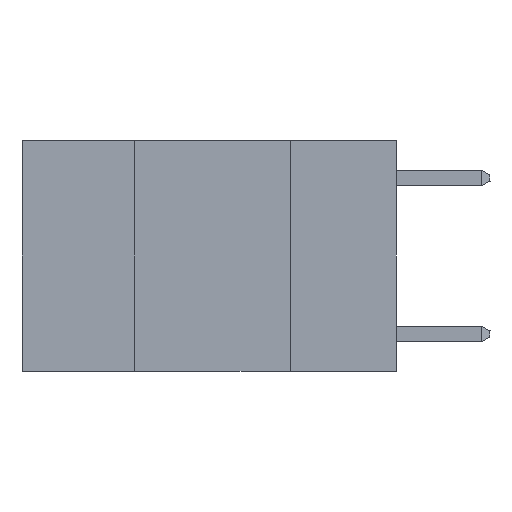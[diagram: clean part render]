
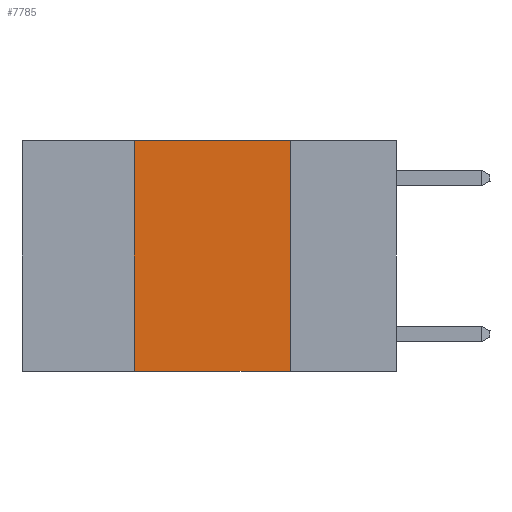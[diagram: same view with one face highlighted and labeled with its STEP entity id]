
A CAD part, left-side view. The second image highlights one B-rep face of the part: STEP entity #7785.
In plain terms, the highlighted planar face has unit normal (-1, 0, 0).
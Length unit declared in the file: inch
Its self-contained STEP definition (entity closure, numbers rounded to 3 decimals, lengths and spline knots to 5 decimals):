
#17 = VERTEX_POINT ( 'NONE', #8199 ) ;
#267 = PLANE ( 'NONE',  #1084 ) ;
#646 = EDGE_CURVE ( 'NONE', #10710, #13058, #12916, .T. ) ;
#807 = CARTESIAN_POINT ( 'NONE',  ( 0., 0.17, 0. ) ) ;
#955 = VECTOR ( 'NONE', #2615, 39.37008 ) ;
#989 = EDGE_CURVE ( 'NONE', #13058, #6762, #6658, .T. ) ;
#1084 = AXIS2_PLACEMENT_3D ( 'NONE', #8690, #9855, #2720 ) ;
#2025 = DIRECTION ( 'NONE',  ( 0., 0., -1. ) ) ;
#2289 = EDGE_CURVE ( 'NONE', #10710, #17, #6254, .T. ) ;
#2615 = DIRECTION ( 'NONE',  ( 0., -1., 0. ) ) ;
#2720 = DIRECTION ( 'NONE',  ( 0., 0., -1. ) ) ;
#2868 = VECTOR ( 'NONE', #7105, 39.37008 ) ;
#3049 = FACE_OUTER_BOUND ( 'NONE', #4966, .T. ) ;
#3768 = VECTOR ( 'NONE', #9450, 39.37008 ) ;
#3850 = CARTESIAN_POINT ( 'NONE',  ( 0., 0.42, 0. ) ) ;
#4619 = CARTESIAN_POINT ( 'NONE',  ( 0., 0.6, -0.37 ) ) ;
#4966 = EDGE_LOOP ( 'NONE', ( #12845, #11351, #13633, #12426 ) ) ;
#6254 = LINE ( 'NONE', #4619, #955 ) ;
#6658 = LINE ( 'NONE', #10931, #2868 ) ;
#6762 = VERTEX_POINT ( 'NONE', #9344 ) ;
#6813 = VECTOR ( 'NONE', #2025, 39.37008 ) ;
#7032 = CARTESIAN_POINT ( 'NONE',  ( 0., 0.42, -0.37 ) ) ;
#7105 = DIRECTION ( 'NONE',  ( 0., -1., 0. ) ) ;
#7785 = ADVANCED_FACE ( 'NONE', ( #3049 ), #267, .F. ) ;
#8092 = CARTESIAN_POINT ( 'NONE',  ( 0., 0.42, 0. ) ) ;
#8199 = CARTESIAN_POINT ( 'NONE',  ( 0., 0.17, -0.37 ) ) ;
#8690 = CARTESIAN_POINT ( 'NONE',  ( 0., 0.6, 0. ) ) ;
#8698 = EDGE_CURVE ( 'NONE', #6762, #17, #13298, .T. ) ;
#9344 = CARTESIAN_POINT ( 'NONE',  ( 0., 0.17, 0. ) ) ;
#9450 = DIRECTION ( 'NONE',  ( 0., 0., 1. ) ) ;
#9855 = DIRECTION ( 'NONE',  ( 1., 0., 0. ) ) ;
#10710 = VERTEX_POINT ( 'NONE', #7032 ) ;
#10931 = CARTESIAN_POINT ( 'NONE',  ( 0., 0.6, 0. ) ) ;
#11351 = ORIENTED_EDGE ( 'NONE', *, *, #989, .F. ) ;
#12426 = ORIENTED_EDGE ( 'NONE', *, *, #2289, .T. ) ;
#12845 = ORIENTED_EDGE ( 'NONE', *, *, #8698, .F. ) ;
#12916 = LINE ( 'NONE', #3850, #3768 ) ;
#13058 = VERTEX_POINT ( 'NONE', #8092 ) ;
#13298 = LINE ( 'NONE', #807, #6813 ) ;
#13633 = ORIENTED_EDGE ( 'NONE', *, *, #646, .F. ) ;
